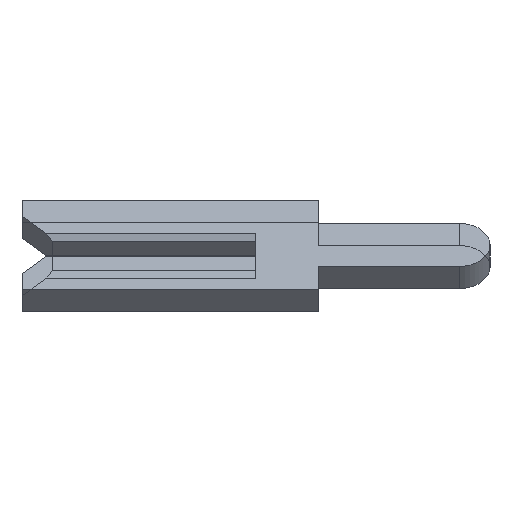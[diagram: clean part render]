
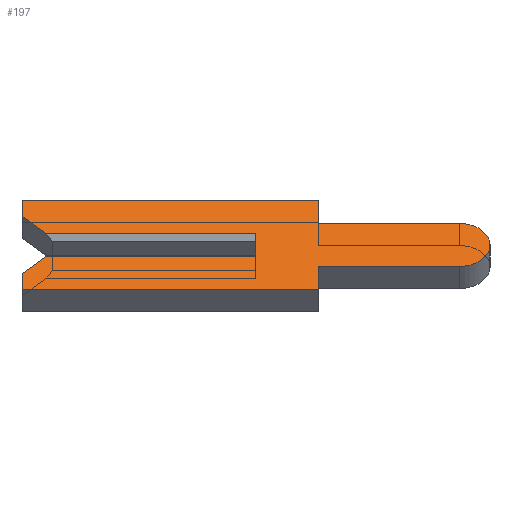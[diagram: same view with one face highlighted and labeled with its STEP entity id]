
A CAD part, left-side view. The second image highlights one B-rep face of the part: STEP entity #197.
In plain terms, the highlighted face is planar.
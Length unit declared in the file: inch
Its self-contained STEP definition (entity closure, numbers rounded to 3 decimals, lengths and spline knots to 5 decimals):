
#17 = DIRECTION ( 'NONE',  ( 0., -1., 0. ) ) ;
#89 = EDGE_CURVE ( 'NONE', #1832, #334, #1375, .T. ) ;
#145 = VERTEX_POINT ( 'NONE', #2450 ) ;
#196 = CARTESIAN_POINT ( 'NONE',  ( -0.01, 0.15, 0.026 ) ) ;
#197 = ADVANCED_FACE ( 'NONE', ( #1611 ), #513, .F. ) ;
#208 = LINE ( 'NONE', #2059, #3079 ) ;
#227 = VECTOR ( 'NONE', #1870, 39.37008 ) ;
#249 = VERTEX_POINT ( 'NONE', #1059 ) ;
#310 = EDGE_CURVE ( 'NONE', #145, #2698, #1428, .T. ) ;
#333 = CARTESIAN_POINT ( 'NONE',  ( -0.01, 0.15, 0.04 ) ) ;
#334 = VERTEX_POINT ( 'NONE', #1089 ) ;
#382 = LINE ( 'NONE', #1117, #594 ) ;
#386 = CARTESIAN_POINT ( 'NONE',  ( -0.01, 0., 0.01 ) ) ;
#401 = DIRECTION ( 'NONE',  ( 0., -1., 0. ) ) ;
#451 = ORIENTED_EDGE ( 'NONE', *, *, #2981, .F. ) ;
#462 = CARTESIAN_POINT ( 'NONE',  ( -0.01, -0.04, 0.04 ) ) ;
#490 = DIRECTION ( 'NONE',  ( 0., 0., -1. ) ) ;
#504 = VECTOR ( 'NONE', #2205, 39.37008 ) ;
#506 = EDGE_CURVE ( 'NONE', #334, #1006, #3374, .T. ) ;
#512 = LINE ( 'NONE', #3341, #1535 ) ;
#513 = PLANE ( 'NONE',  #1444 ) ;
#531 = VECTOR ( 'NONE', #401, 39.37008 ) ;
#546 = EDGE_CURVE ( 'NONE', #2222, #692, #512, .T. ) ;
#554 = ORIENTED_EDGE ( 'NONE', *, *, #2058, .F. ) ;
#594 = VECTOR ( 'NONE', #1394, 39.37008 ) ;
#621 = EDGE_CURVE ( 'NONE', #2698, #249, #2100, .T. ) ;
#628 = VECTOR ( 'NONE', #2724, 39.37008 ) ;
#644 = VERTEX_POINT ( 'NONE', #2507 ) ;
#674 = CIRCLE ( 'NONE', #3087, 0.0195 ) ;
#691 = LINE ( 'NONE', #854, #2332 ) ;
#692 = VERTEX_POINT ( 'NONE', #2778 ) ;
#774 = CARTESIAN_POINT ( 'NONE',  ( -0.01, 0.1305, -0.0065 ) ) ;
#817 = EDGE_CURVE ( 'NONE', #1006, #2208, #382, .T. ) ;
#854 = CARTESIAN_POINT ( 'NONE',  ( -0.01, 0.15, 0.01 ) ) ;
#866 = DIRECTION ( 'NONE',  ( 0., -1., 0. ) ) ;
#880 = EDGE_CURVE ( 'NONE', #2141, #2208, #691, .T. ) ;
#896 = ORIENTED_EDGE ( 'NONE', *, *, #621, .F. ) ;
#909 = CARTESIAN_POINT ( 'NONE',  ( -0.01, -0.1305, 0. ) ) ;
#935 = EDGE_CURVE ( 'NONE', #2141, #2297, #2738, .T. ) ;
#1006 = VERTEX_POINT ( 'NONE', #1386 ) ;
#1009 = ORIENTED_EDGE ( 'NONE', *, *, #89, .F. ) ;
#1059 = CARTESIAN_POINT ( 'NONE',  ( -0.01, 0.15, -0.04 ) ) ;
#1089 = CARTESIAN_POINT ( 'NONE',  ( -0.01, 0.134, -0.01 ) ) ;
#1093 = ORIENTED_EDGE ( 'NONE', *, *, #3294, .F. ) ;
#1117 = CARTESIAN_POINT ( 'NONE',  ( -0.01, 0., 0.0065 ) ) ;
#1149 = LINE ( 'NONE', #462, #1725 ) ;
#1157 = EDGE_LOOP ( 'NONE', ( #2519, #2185, #2859, #1009, #3302, #896, #2446, #2575, #2311, #3040, #1093, #554, #451, #3000 ) ) ;
#1187 = DIRECTION ( 'NONE',  ( 1., 0., 0. ) ) ;
#1262 = VECTOR ( 'NONE', #2248, 39.37008 ) ;
#1307 = EDGE_CURVE ( 'NONE', #249, #1832, #208, .T. ) ;
#1375 = LINE ( 'NONE', #774, #628 ) ;
#1386 = CARTESIAN_POINT ( 'NONE',  ( -0.01, 0., -0.01 ) ) ;
#1394 = DIRECTION ( 'NONE',  ( 0., 0., 1. ) ) ;
#1405 = CARTESIAN_POINT ( 'NONE',  ( -0.01, 0.1305, 0.0065 ) ) ;
#1419 = DIRECTION ( 'NONE',  ( 0., 0.707, 0.707 ) ) ;
#1428 = LINE ( 'NONE', #2770, #504 ) ;
#1444 = AXIS2_PLACEMENT_3D ( 'NONE', #1621, #2481, #490 ) ;
#1445 = CARTESIAN_POINT ( 'NONE',  ( -0.01, 0.15, -0.026 ) ) ;
#1478 = CARTESIAN_POINT ( 'NONE',  ( -0.01, 0.15, 0.04 ) ) ;
#1535 = VECTOR ( 'NONE', #866, 39.37008 ) ;
#1539 = CARTESIAN_POINT ( 'NONE',  ( -0.01, 0.15, 0.026 ) ) ;
#1611 = FACE_OUTER_BOUND ( 'NONE', #1157, .T. ) ;
#1621 = CARTESIAN_POINT ( 'NONE',  ( -0.01, -0.1305, 0. ) ) ;
#1725 = VECTOR ( 'NONE', #2983, 39.37008 ) ;
#1818 = CARTESIAN_POINT ( 'NONE',  ( -0.01, -0.04, -0.04 ) ) ;
#1832 = VERTEX_POINT ( 'NONE', #1445 ) ;
#1868 = EDGE_CURVE ( 'NONE', #692, #644, #674, .T. ) ;
#1870 = DIRECTION ( 'NONE',  ( 0., 0., 1. ) ) ;
#1894 = LINE ( 'NONE', #196, #227 ) ;
#1934 = EDGE_CURVE ( 'NONE', #644, #145, #2080, .T. ) ;
#1995 = DIRECTION ( 'NONE',  ( 0., -1., 0. ) ) ;
#2005 = VERTEX_POINT ( 'NONE', #1478 ) ;
#2007 = DIRECTION ( 'NONE',  ( 0., 0., 1. ) ) ;
#2058 = EDGE_CURVE ( 'NONE', #2005, #3214, #2381, .T. ) ;
#2059 = CARTESIAN_POINT ( 'NONE',  ( -0.01, 0.15, -0.026 ) ) ;
#2080 = LINE ( 'NONE', #3419, #3272 ) ;
#2100 = LINE ( 'NONE', #2237, #1262 ) ;
#2141 = VERTEX_POINT ( 'NONE', #2325 ) ;
#2185 = ORIENTED_EDGE ( 'NONE', *, *, #817, .F. ) ;
#2205 = DIRECTION ( 'NONE',  ( 0., 0., -1. ) ) ;
#2208 = VERTEX_POINT ( 'NONE', #386 ) ;
#2222 = VERTEX_POINT ( 'NONE', #3439 ) ;
#2237 = CARTESIAN_POINT ( 'NONE',  ( -0.01, 0.15, -0.04 ) ) ;
#2248 = DIRECTION ( 'NONE',  ( 0., 1., 0. ) ) ;
#2256 = CARTESIAN_POINT ( 'NONE',  ( -0.01, -0.1305, -0.01 ) ) ;
#2297 = VERTEX_POINT ( 'NONE', #1539 ) ;
#2311 = ORIENTED_EDGE ( 'NONE', *, *, #1868, .F. ) ;
#2325 = CARTESIAN_POINT ( 'NONE',  ( -0.01, 0.134, 0.01 ) ) ;
#2332 = VECTOR ( 'NONE', #1995, 39.37008 ) ;
#2381 = LINE ( 'NONE', #333, #531 ) ;
#2442 = VECTOR ( 'NONE', #1419, 39.37008 ) ;
#2446 = ORIENTED_EDGE ( 'NONE', *, *, #310, .F. ) ;
#2450 = CARTESIAN_POINT ( 'NONE',  ( -0.01, -0.04, -0.0195 ) ) ;
#2481 = DIRECTION ( 'NONE',  ( 1., 0., 0. ) ) ;
#2507 = CARTESIAN_POINT ( 'NONE',  ( -0.01, -0.1305, -0.0195 ) ) ;
#2519 = ORIENTED_EDGE ( 'NONE', *, *, #880, .T. ) ;
#2575 = ORIENTED_EDGE ( 'NONE', *, *, #1934, .F. ) ;
#2698 = VERTEX_POINT ( 'NONE', #1818 ) ;
#2720 = CARTESIAN_POINT ( 'NONE',  ( -0.01, -0.04, 0.04 ) ) ;
#2724 = DIRECTION ( 'NONE',  ( 0., -0.707, 0.707 ) ) ;
#2738 = LINE ( 'NONE', #1405, #2442 ) ;
#2770 = CARTESIAN_POINT ( 'NONE',  ( -0.01, -0.04, -0.04 ) ) ;
#2778 = CARTESIAN_POINT ( 'NONE',  ( -0.01, -0.1305, 0.0195 ) ) ;
#2820 = VECTOR ( 'NONE', #17, 39.37008 ) ;
#2859 = ORIENTED_EDGE ( 'NONE', *, *, #506, .F. ) ;
#2981 = EDGE_CURVE ( 'NONE', #2297, #2005, #1894, .T. ) ;
#2983 = DIRECTION ( 'NONE',  ( 0., 0., -1. ) ) ;
#3000 = ORIENTED_EDGE ( 'NONE', *, *, #935, .F. ) ;
#3040 = ORIENTED_EDGE ( 'NONE', *, *, #546, .F. ) ;
#3079 = VECTOR ( 'NONE', #2007, 39.37008 ) ;
#3087 = AXIS2_PLACEMENT_3D ( 'NONE', #909, #1187, #3134 ) ;
#3101 = DIRECTION ( 'NONE',  ( 0., 1., 0. ) ) ;
#3134 = DIRECTION ( 'NONE',  ( 0., 0., -1. ) ) ;
#3214 = VERTEX_POINT ( 'NONE', #2720 ) ;
#3272 = VECTOR ( 'NONE', #3101, 39.37008 ) ;
#3294 = EDGE_CURVE ( 'NONE', #3214, #2222, #1149, .T. ) ;
#3302 = ORIENTED_EDGE ( 'NONE', *, *, #1307, .F. ) ;
#3341 = CARTESIAN_POINT ( 'NONE',  ( -0.01, -0.04, 0.0195 ) ) ;
#3374 = LINE ( 'NONE', #2256, #2820 ) ;
#3419 = CARTESIAN_POINT ( 'NONE',  ( -0.01, -0.04, -0.0195 ) ) ;
#3439 = CARTESIAN_POINT ( 'NONE',  ( -0.01, -0.04, 0.0195 ) ) ;
